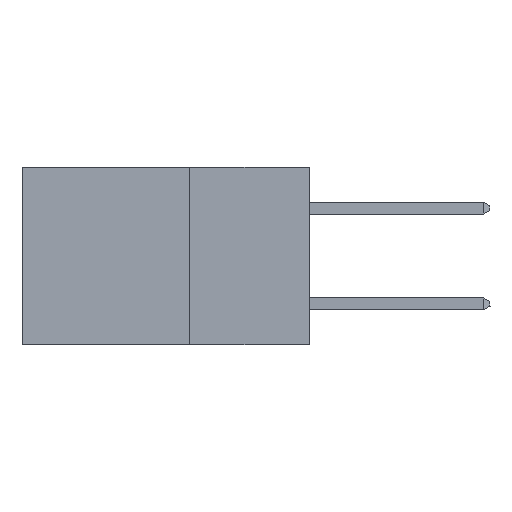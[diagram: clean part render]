
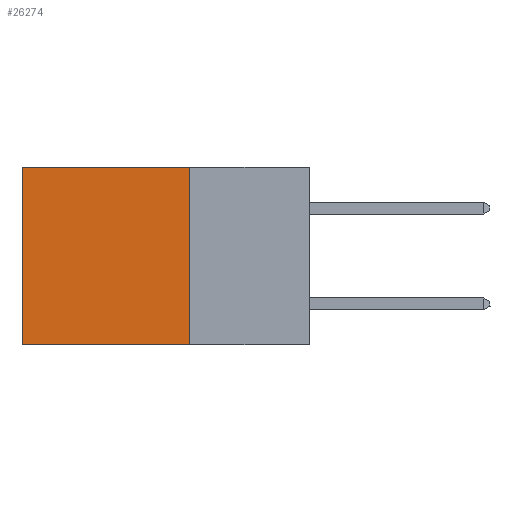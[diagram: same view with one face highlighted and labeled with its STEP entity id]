
A CAD part, left-side view. The second image highlights one B-rep face of the part: STEP entity #26274.
In plain terms, the highlighted planar face has unit normal (-1, 0, 0).
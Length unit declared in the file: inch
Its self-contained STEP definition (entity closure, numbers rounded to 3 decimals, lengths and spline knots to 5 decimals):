
#277 = CARTESIAN_POINT ( 'NONE',  ( 0.2875, 0.25, -0.37 ) ) ;
#426 = LINE ( 'NONE', #21004, #15514 ) ;
#1739 = ORIENTED_EDGE ( 'NONE', *, *, #20411, .T. ) ;
#2284 = DIRECTION ( 'NONE',  ( 1., 0., 0. ) ) ;
#2476 = LINE ( 'NONE', #15866, #2796 ) ;
#2565 = AXIS2_PLACEMENT_3D ( 'NONE', #8648, #2284, #12671 ) ;
#2796 = VECTOR ( 'NONE', #11819, 39.37008 ) ;
#4929 = FACE_OUTER_BOUND ( 'NONE', #7430, .T. ) ;
#5236 = LINE ( 'NONE', #9935, #5922 ) ;
#5922 = VECTOR ( 'NONE', #26923, 39.37008 ) ;
#5962 = CARTESIAN_POINT ( 'NONE',  ( 0.2875, 0.6, 0. ) ) ;
#7430 = EDGE_LOOP ( 'NONE', ( #19129, #17013, #26098, #1739 ) ) ;
#7455 = VERTEX_POINT ( 'NONE', #18279 ) ;
#8232 = DIRECTION ( 'NONE',  ( 0., 1., 0. ) ) ;
#8648 = CARTESIAN_POINT ( 'NONE',  ( 0.2875, 0.25, 0. ) ) ;
#9173 = VERTEX_POINT ( 'NONE', #277 ) ;
#9935 = CARTESIAN_POINT ( 'NONE',  ( 0.2875, 0.6, 0. ) ) ;
#11456 = EDGE_CURVE ( 'NONE', #9173, #13366, #26787, .T. ) ;
#11819 = DIRECTION ( 'NONE',  ( 0., 0., -1. ) ) ;
#12671 = DIRECTION ( 'NONE',  ( 0., 0., -1. ) ) ;
#13366 = VERTEX_POINT ( 'NONE', #23477 ) ;
#15514 = VECTOR ( 'NONE', #8232, 39.37008 ) ;
#15866 = CARTESIAN_POINT ( 'NONE',  ( 0.2875, 0.25, 0. ) ) ;
#17013 = ORIENTED_EDGE ( 'NONE', *, *, #11456, .F. ) ;
#17729 = VECTOR ( 'NONE', #21500, 39.37008 ) ;
#18279 = CARTESIAN_POINT ( 'NONE',  ( 0.2875, 0.25, 0. ) ) ;
#19129 = ORIENTED_EDGE ( 'NONE', *, *, #26608, .T. ) ;
#19347 = PLANE ( 'NONE',  #2565 ) ;
#20094 = EDGE_CURVE ( 'NONE', #7455, #9173, #2476, .T. ) ;
#20411 = EDGE_CURVE ( 'NONE', #7455, #23102, #426, .T. ) ;
#21004 = CARTESIAN_POINT ( 'NONE',  ( 0.2875, 0.25, 0. ) ) ;
#21500 = DIRECTION ( 'NONE',  ( 0., 1., 0. ) ) ;
#23102 = VERTEX_POINT ( 'NONE', #5962 ) ;
#23477 = CARTESIAN_POINT ( 'NONE',  ( 0.2875, 0.6, -0.37 ) ) ;
#25531 = CARTESIAN_POINT ( 'NONE',  ( 0.2875, 0.25, -0.37 ) ) ;
#26098 = ORIENTED_EDGE ( 'NONE', *, *, #20094, .F. ) ;
#26274 = ADVANCED_FACE ( 'NONE', ( #4929 ), #19347, .F. ) ;
#26608 = EDGE_CURVE ( 'NONE', #23102, #13366, #5236, .T. ) ;
#26787 = LINE ( 'NONE', #25531, #17729 ) ;
#26923 = DIRECTION ( 'NONE',  ( 0., 0., -1. ) ) ;
